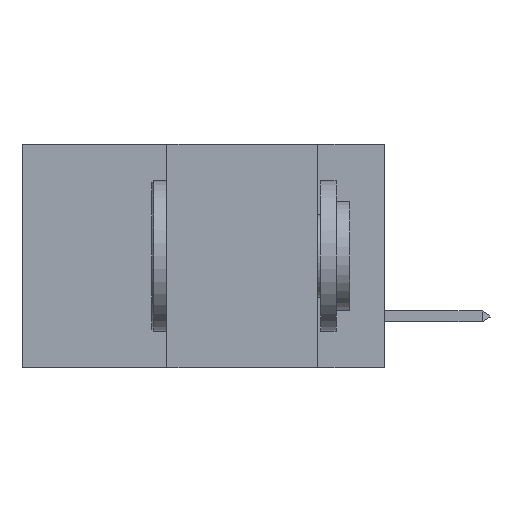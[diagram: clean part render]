
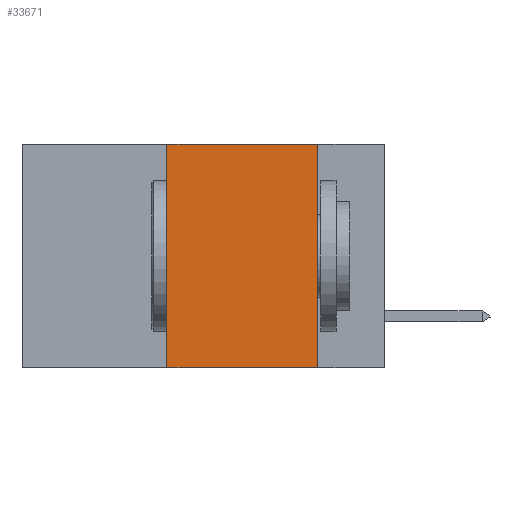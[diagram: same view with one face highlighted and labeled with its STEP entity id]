
A CAD part, left-side view. The second image highlights one B-rep face of the part: STEP entity #33671.
In plain terms, the highlighted planar face has unit normal (-1, 0, 0).
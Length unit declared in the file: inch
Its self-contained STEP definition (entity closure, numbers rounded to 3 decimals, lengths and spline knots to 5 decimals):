
#1826 = ORIENTED_EDGE ( 'NONE', *, *, #2278, .F. ) ;
#2278 = EDGE_CURVE ( 'NONE', #12709, #41400, #17604, .T. ) ;
#2847 = CARTESIAN_POINT ( 'NONE',  ( 0., 0.36, -0.37 ) ) ;
#4244 = DIRECTION ( 'NONE',  ( 0., 0., 1. ) ) ;
#4505 = VECTOR ( 'NONE', #4244, 39.37008 ) ;
#6080 = DIRECTION ( 'NONE',  ( 0., -1., 0. ) ) ;
#6799 = LINE ( 'NONE', #19872, #19308 ) ;
#7882 = EDGE_CURVE ( 'NONE', #17667, #34532, #13741, .T. ) ;
#11470 = ORIENTED_EDGE ( 'NONE', *, *, #22407, .F. ) ;
#12709 = VERTEX_POINT ( 'NONE', #27268 ) ;
#13013 = CARTESIAN_POINT ( 'NONE',  ( 0., 0.11, 0. ) ) ;
#13741 = LINE ( 'NONE', #15272, #4505 ) ;
#14604 = CARTESIAN_POINT ( 'NONE',  ( 0., 0.36, 0. ) ) ;
#15219 = ORIENTED_EDGE ( 'NONE', *, *, #7882, .F. ) ;
#15272 = CARTESIAN_POINT ( 'NONE',  ( 0., 0.36, 0. ) ) ;
#16423 = LINE ( 'NONE', #24208, #26029 ) ;
#17604 = LINE ( 'NONE', #13013, #34032 ) ;
#17667 = VERTEX_POINT ( 'NONE', #2847 ) ;
#18792 = CARTESIAN_POINT ( 'NONE',  ( 0., 0.11, -0.37 ) ) ;
#18802 = FACE_OUTER_BOUND ( 'NONE', #23202, .T. ) ;
#19308 = VECTOR ( 'NONE', #42016, 39.37008 ) ;
#19843 = DIRECTION ( 'NONE',  ( 0., 0., -1. ) ) ;
#19872 = CARTESIAN_POINT ( 'NONE',  ( 0., 0.6, -0.37 ) ) ;
#22407 = EDGE_CURVE ( 'NONE', #34532, #12709, #16423, .T. ) ;
#23202 = EDGE_LOOP ( 'NONE', ( #1826, #11470, #15219, #31102 ) ) ;
#24208 = CARTESIAN_POINT ( 'NONE',  ( 0., 0.6, 0. ) ) ;
#26029 = VECTOR ( 'NONE', #6080, 39.37008 ) ;
#26725 = DIRECTION ( 'NONE',  ( 1., 0., 0. ) ) ;
#27268 = CARTESIAN_POINT ( 'NONE',  ( 0., 0.11, 0. ) ) ;
#28578 = AXIS2_PLACEMENT_3D ( 'NONE', #45576, #26725, #31032 ) ;
#31032 = DIRECTION ( 'NONE',  ( 0., 0., -1. ) ) ;
#31102 = ORIENTED_EDGE ( 'NONE', *, *, #38381, .T. ) ;
#33671 = ADVANCED_FACE ( 'NONE', ( #18802 ), #34218, .F. ) ;
#34032 = VECTOR ( 'NONE', #19843, 39.37008 ) ;
#34218 = PLANE ( 'NONE',  #28578 ) ;
#34532 = VERTEX_POINT ( 'NONE', #14604 ) ;
#38381 = EDGE_CURVE ( 'NONE', #17667, #41400, #6799, .T. ) ;
#41400 = VERTEX_POINT ( 'NONE', #18792 ) ;
#42016 = DIRECTION ( 'NONE',  ( 0., -1., 0. ) ) ;
#45576 = CARTESIAN_POINT ( 'NONE',  ( 0., 0.6, 0. ) ) ;
